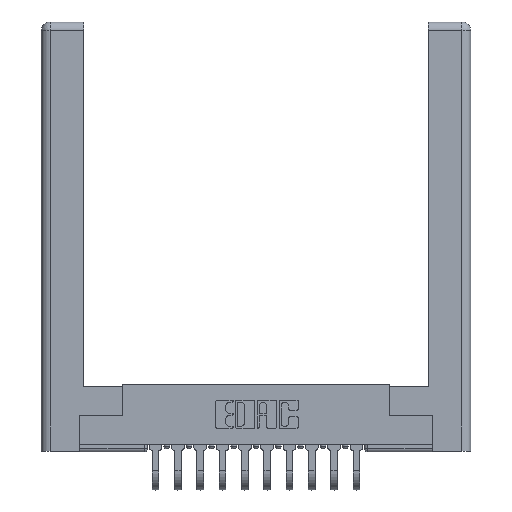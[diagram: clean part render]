
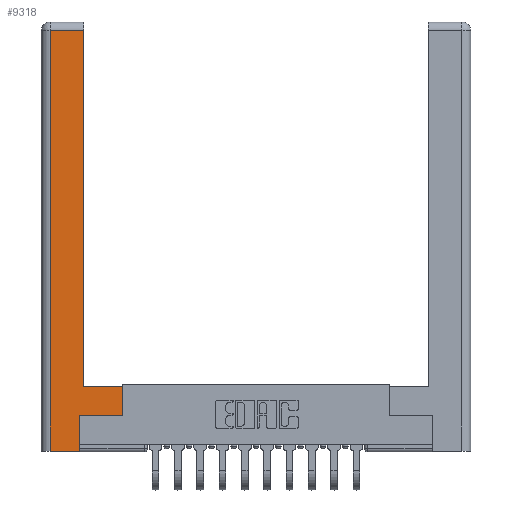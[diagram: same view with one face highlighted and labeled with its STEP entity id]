
A CAD part, top view. The second image highlights one B-rep face of the part: STEP entity #9318.
In plain terms, the highlighted planar face has unit normal (0, 0, 1).
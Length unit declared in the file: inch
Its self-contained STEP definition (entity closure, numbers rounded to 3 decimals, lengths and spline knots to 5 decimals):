
#72 = EDGE_CURVE ( 'NONE', #10490, #11538, #15252, .T. ) ;
#145 = VECTOR ( 'NONE', #6606, 39.37008 ) ;
#610 = VERTEX_POINT ( 'NONE', #5022 ) ;
#612 = ORIENTED_EDGE ( 'NONE', *, *, #72, .T. ) ;
#942 = VECTOR ( 'NONE', #2271, 39.37008 ) ;
#1041 = CARTESIAN_POINT ( 'NONE',  ( 0.0615, 2.94, 0. ) ) ;
#1100 = VECTOR ( 'NONE', #4376, 39.37008 ) ;
#1273 = EDGE_CURVE ( 'NONE', #4117, #610, #8706, .T. ) ;
#1348 = EDGE_CURVE ( 'NONE', #14890, #4522, #15044, .T. ) ;
#1824 = VERTEX_POINT ( 'NONE', #4568 ) ;
#2235 = DIRECTION ( 'NONE',  ( 0., 1., 0. ) ) ;
#2270 = EDGE_CURVE ( 'NONE', #10610, #14890, #9409, .T. ) ;
#2271 = DIRECTION ( 'NONE',  ( 0., 1., 0. ) ) ;
#2413 = ORIENTED_EDGE ( 'NONE', *, *, #8363, .T. ) ;
#3004 = LINE ( 'NONE', #13423, #8187 ) ;
#3418 = DIRECTION ( 'NONE',  ( 1., 0., 0. ) ) ;
#4117 = VERTEX_POINT ( 'NONE', #10926 ) ;
#4376 = DIRECTION ( 'NONE',  ( 1., 0., 0. ) ) ;
#4522 = VERTEX_POINT ( 'NONE', #6579 ) ;
#4568 = CARTESIAN_POINT ( 'NONE',  ( 0.565, 0.45, 0. ) ) ;
#4612 = LINE ( 'NONE', #9618, #12065 ) ;
#5022 = CARTESIAN_POINT ( 'NONE',  ( 0.0615, 0., 0. ) ) ;
#5207 = CARTESIAN_POINT ( 'NONE',  ( 0., 0., 0. ) ) ;
#5628 = EDGE_CURVE ( 'NONE', #4522, #1824, #4612, .T. ) ;
#5986 = DIRECTION ( 'NONE',  ( 0., 1., 0. ) ) ;
#6579 = CARTESIAN_POINT ( 'NONE',  ( 0.565, 0.245, 0. ) ) ;
#6606 = DIRECTION ( 'NONE',  ( 0., -1., 0. ) ) ;
#6722 = ORIENTED_EDGE ( 'NONE', *, *, #5628, .T. ) ;
#6911 = CARTESIAN_POINT ( 'NONE',  ( 0.565, 0.245, 0. ) ) ;
#6962 = CARTESIAN_POINT ( 'NONE',  ( 0.265, 0., 0. ) ) ;
#7168 = ORIENTED_EDGE ( 'NONE', *, *, #1273, .T. ) ;
#7633 = CARTESIAN_POINT ( 'NONE',  ( 0.295, 2.94, 0. ) ) ;
#7728 = CARTESIAN_POINT ( 'NONE',  ( 0.265, 0.245, 0. ) ) ;
#7832 = EDGE_CURVE ( 'NONE', #610, #10610, #8199, .T. ) ;
#8187 = VECTOR ( 'NONE', #12419, 39.37008 ) ;
#8199 = LINE ( 'NONE', #6962, #11872 ) ;
#8363 = EDGE_CURVE ( 'NONE', #1824, #10490, #3004, .T. ) ;
#8443 = DIRECTION ( 'NONE',  ( -1., 0., 0. ) ) ;
#8706 = LINE ( 'NONE', #13639, #145 ) ;
#9135 = LINE ( 'NONE', #1041, #14653 ) ;
#9318 = ADVANCED_FACE ( 'NONE', ( #9753 ), #13308, .F. ) ;
#9369 = EDGE_LOOP ( 'NONE', ( #612, #11023, #7168, #14090, #11601, #14275, #6722, #2413 ) ) ;
#9373 = VECTOR ( 'NONE', #2235, 39.37008 ) ;
#9409 = LINE ( 'NONE', #14041, #9373 ) ;
#9618 = CARTESIAN_POINT ( 'NONE',  ( 0.565, 0.45, 0. ) ) ;
#9753 = FACE_OUTER_BOUND ( 'NONE', #9369, .T. ) ;
#10054 = CARTESIAN_POINT ( 'NONE',  ( 0.265, 0., 0. ) ) ;
#10490 = VERTEX_POINT ( 'NONE', #10992 ) ;
#10610 = VERTEX_POINT ( 'NONE', #10054 ) ;
#10926 = CARTESIAN_POINT ( 'NONE',  ( 0.0615, 2.94, 0. ) ) ;
#10992 = CARTESIAN_POINT ( 'NONE',  ( 0.295, 0.45, 0. ) ) ;
#11023 = ORIENTED_EDGE ( 'NONE', *, *, #14646, .T. ) ;
#11538 = VERTEX_POINT ( 'NONE', #7633 ) ;
#11601 = ORIENTED_EDGE ( 'NONE', *, *, #2270, .T. ) ;
#11872 = VECTOR ( 'NONE', #3418, 39.37008 ) ;
#12065 = VECTOR ( 'NONE', #5986, 39.37008 ) ;
#12419 = DIRECTION ( 'NONE',  ( -1., 0., 0. ) ) ;
#12976 = AXIS2_PLACEMENT_3D ( 'NONE', #5207, #13464, #8443 ) ;
#13308 = PLANE ( 'NONE',  #12976 ) ;
#13423 = CARTESIAN_POINT ( 'NONE',  ( 0.295, 0.45, 0. ) ) ;
#13464 = DIRECTION ( 'NONE',  ( 0., 0., -1. ) ) ;
#13639 = CARTESIAN_POINT ( 'NONE',  ( 0.0615, 0., 0. ) ) ;
#13925 = CARTESIAN_POINT ( 'NONE',  ( 0.295, 3., 0. ) ) ;
#14041 = CARTESIAN_POINT ( 'NONE',  ( 0.265, 0.245, 0. ) ) ;
#14090 = ORIENTED_EDGE ( 'NONE', *, *, #7832, .T. ) ;
#14275 = ORIENTED_EDGE ( 'NONE', *, *, #1348, .T. ) ;
#14646 = EDGE_CURVE ( 'NONE', #11538, #4117, #9135, .T. ) ;
#14653 = VECTOR ( 'NONE', #15103, 39.37008 ) ;
#14890 = VERTEX_POINT ( 'NONE', #7728 ) ;
#15044 = LINE ( 'NONE', #6911, #1100 ) ;
#15103 = DIRECTION ( 'NONE',  ( -1., 0., 0. ) ) ;
#15252 = LINE ( 'NONE', #13925, #942 ) ;
